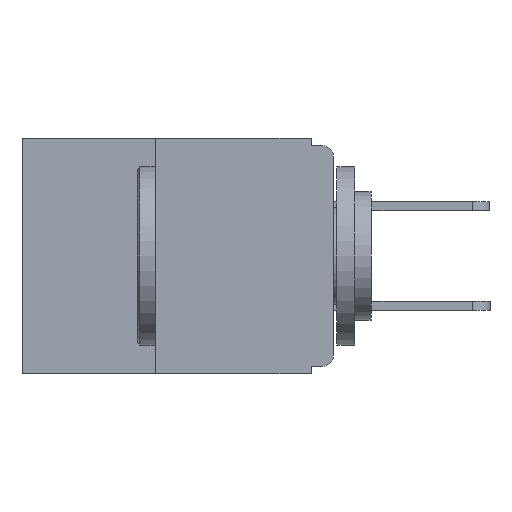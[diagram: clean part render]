
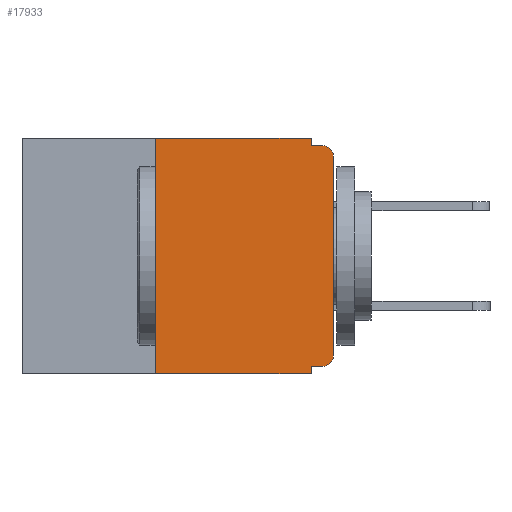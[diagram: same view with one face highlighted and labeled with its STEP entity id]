
A CAD part, left-side view. The second image highlights one B-rep face of the part: STEP entity #17933.
In plain terms, the highlighted planar face has unit normal (-1, 0, 0).
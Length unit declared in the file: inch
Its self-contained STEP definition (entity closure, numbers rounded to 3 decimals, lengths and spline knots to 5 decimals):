
#354 = VERTEX_POINT ( 'NONE', #6901 ) ;
#371 = LINE ( 'NONE', #10115, #14249 ) ;
#398 = CIRCLE ( 'NONE', #11670, 0.015 ) ;
#417 = DIRECTION ( 'NONE',  ( 0., 0., -1. ) ) ;
#419 = DIRECTION ( 'NONE',  ( -1., 0., 0. ) ) ;
#480 = CARTESIAN_POINT ( 'NONE',  ( 0., 0.015, -0.025 ) ) ;
#1076 = ORIENTED_EDGE ( 'NONE', *, *, #2373, .T. ) ;
#1140 = VERTEX_POINT ( 'NONE', #5741 ) ;
#1187 = VERTEX_POINT ( 'NONE', #22572 ) ;
#1360 = CARTESIAN_POINT ( 'NONE',  ( 0., 0., -0.305 ) ) ;
#1577 = VECTOR ( 'NONE', #4752, 39.37008 ) ;
#1814 = VERTEX_POINT ( 'NONE', #17164 ) ;
#1894 = LINE ( 'NONE', #11951, #19674 ) ;
#1923 = VECTOR ( 'NONE', #22673, 39.37008 ) ;
#1949 = ORIENTED_EDGE ( 'NONE', *, *, #7261, .F. ) ;
#2303 = VERTEX_POINT ( 'NONE', #5674 ) ;
#2373 = EDGE_CURVE ( 'NONE', #1140, #21010, #18681, .T. ) ;
#2785 = DIRECTION ( 'NONE',  ( 0., -1., 0. ) ) ;
#2897 = CARTESIAN_POINT ( 'NONE',  ( 0., 0.437, -0.33 ) ) ;
#3483 = CARTESIAN_POINT ( 'NONE',  ( 0., 0., -0.01 ) ) ;
#3536 = DIRECTION ( 'NONE',  ( 0., -1., 0. ) ) ;
#3557 = EDGE_CURVE ( 'NONE', #1814, #354, #15412, .T. ) ;
#3966 = LINE ( 'NONE', #14032, #21945 ) ;
#4752 = DIRECTION ( 'NONE',  ( 0., -1., 0. ) ) ;
#5023 = EDGE_CURVE ( 'NONE', #16427, #2303, #13108, .T. ) ;
#5286 = CARTESIAN_POINT ( 'NONE',  ( 0., 0.437, 0. ) ) ;
#5674 = CARTESIAN_POINT ( 'NONE',  ( 0., 0.031, -0.32 ) ) ;
#5741 = CARTESIAN_POINT ( 'NONE',  ( 0., 0.25, -0.33 ) ) ;
#6458 = AXIS2_PLACEMENT_3D ( 'NONE', #480, #419, #417 ) ;
#6901 = CARTESIAN_POINT ( 'NONE',  ( 0., 0.031, 0. ) ) ;
#7261 = EDGE_CURVE ( 'NONE', #1140, #1814, #1894, .T. ) ;
#7499 = ORIENTED_EDGE ( 'NONE', *, *, #13103, .T. ) ;
#7907 = CARTESIAN_POINT ( 'NONE',  ( 0., 0.437, 0. ) ) ;
#8109 = CARTESIAN_POINT ( 'NONE',  ( 0., 0., -0.025 ) ) ;
#8452 = EDGE_CURVE ( 'NONE', #354, #1187, #371, .T. ) ;
#8934 = DIRECTION ( 'NONE',  ( 0., 0., -1. ) ) ;
#9108 = ORIENTED_EDGE ( 'NONE', *, *, #14162, .T. ) ;
#9287 = VECTOR ( 'NONE', #3536, 39.37008 ) ;
#9323 = VECTOR ( 'NONE', #2785, 39.37008 ) ;
#9601 = DIRECTION ( 'NONE',  ( -1., 0., 0. ) ) ;
#9722 = DIRECTION ( 'NONE',  ( 0., 0., -1. ) ) ;
#9779 = VERTEX_POINT ( 'NONE', #8109 ) ;
#9853 = LINE ( 'NONE', #3483, #9287 ) ;
#10115 = CARTESIAN_POINT ( 'NONE',  ( 0., 0.031, 0. ) ) ;
#10594 = CARTESIAN_POINT ( 'NONE',  ( 0., 0.031, -0.33 ) ) ;
#11670 = AXIS2_PLACEMENT_3D ( 'NONE', #20014, #9601, #21658 ) ;
#11849 = AXIS2_PLACEMENT_3D ( 'NONE', #7907, #20135, #9722 ) ;
#11951 = CARTESIAN_POINT ( 'NONE',  ( 0., 0.25, -0.33 ) ) ;
#12434 = ORIENTED_EDGE ( 'NONE', *, *, #12957, .F. ) ;
#12442 = ORIENTED_EDGE ( 'NONE', *, *, #5023, .F. ) ;
#12488 = DIRECTION ( 'NONE',  ( 0., 0., 1. ) ) ;
#12558 = VECTOR ( 'NONE', #15154, 39.37008 ) ;
#12957 = EDGE_CURVE ( 'NONE', #1187, #15956, #9853, .T. ) ;
#13062 = ORIENTED_EDGE ( 'NONE', *, *, #22745, .F. ) ;
#13103 = EDGE_CURVE ( 'NONE', #22652, #9779, #16280, .T. ) ;
#13108 = LINE ( 'NONE', #15309, #12558 ) ;
#13158 = FACE_OUTER_BOUND ( 'NONE', #18029, .T. ) ;
#13424 = CARTESIAN_POINT ( 'NONE',  ( 0., 0.015, -0.32 ) ) ;
#13589 = CARTESIAN_POINT ( 'NONE',  ( 0., 0.015, -0.01 ) ) ;
#13603 = CIRCLE ( 'NONE', #6458, 0.015 ) ;
#14032 = CARTESIAN_POINT ( 'NONE',  ( 0., 0.031, -0.33 ) ) ;
#14162 = EDGE_CURVE ( 'NONE', #9779, #15956, #13603, .T. ) ;
#14249 = VECTOR ( 'NONE', #8934, 39.37008 ) ;
#15031 = ORIENTED_EDGE ( 'NONE', *, *, #8452, .F. ) ;
#15154 = DIRECTION ( 'NONE',  ( 0., 1., 0. ) ) ;
#15309 = CARTESIAN_POINT ( 'NONE',  ( 0., 0., -0.32 ) ) ;
#15412 = LINE ( 'NONE', #5286, #1577 ) ;
#15564 = ORIENTED_EDGE ( 'NONE', *, *, #3557, .F. ) ;
#15822 = DIRECTION ( 'NONE',  ( 0., 0., -1. ) ) ;
#15956 = VERTEX_POINT ( 'NONE', #13589 ) ;
#16280 = LINE ( 'NONE', #22624, #1923 ) ;
#16427 = VERTEX_POINT ( 'NONE', #13424 ) ;
#17164 = CARTESIAN_POINT ( 'NONE',  ( 0., 0.25, 0. ) ) ;
#17267 = EDGE_CURVE ( 'NONE', #16427, #22652, #398, .T. ) ;
#17481 = ORIENTED_EDGE ( 'NONE', *, *, #17267, .T. ) ;
#17933 = ADVANCED_FACE ( 'NONE', ( #13158 ), #21631, .F. ) ;
#18029 = EDGE_LOOP ( 'NONE', ( #7499, #9108, #12434, #15031, #15564, #1949, #1076, #13062, #12442, #17481 ) ) ;
#18681 = LINE ( 'NONE', #2897, #9323 ) ;
#19674 = VECTOR ( 'NONE', #12488, 39.37008 ) ;
#20014 = CARTESIAN_POINT ( 'NONE',  ( 0., 0.015, -0.305 ) ) ;
#20135 = DIRECTION ( 'NONE',  ( 1., 0., 0. ) ) ;
#21010 = VERTEX_POINT ( 'NONE', #10594 ) ;
#21631 = PLANE ( 'NONE',  #11849 ) ;
#21658 = DIRECTION ( 'NONE',  ( 0., 0., -1. ) ) ;
#21945 = VECTOR ( 'NONE', #15822, 39.37008 ) ;
#22572 = CARTESIAN_POINT ( 'NONE',  ( 0., 0.031, -0.01 ) ) ;
#22624 = CARTESIAN_POINT ( 'NONE',  ( 0., 0., 0. ) ) ;
#22652 = VERTEX_POINT ( 'NONE', #1360 ) ;
#22673 = DIRECTION ( 'NONE',  ( 0., 0., 1. ) ) ;
#22745 = EDGE_CURVE ( 'NONE', #2303, #21010, #3966, .T. ) ;
